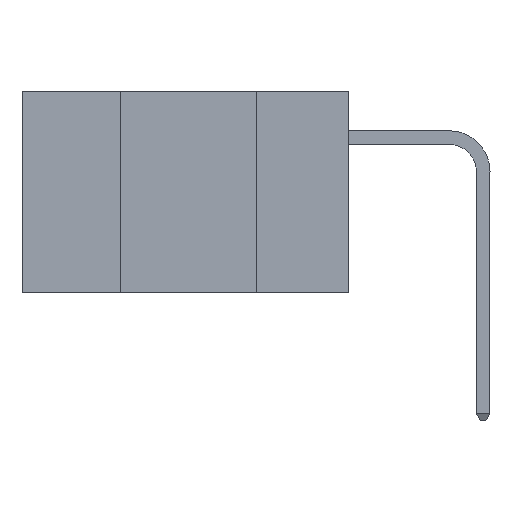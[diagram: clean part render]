
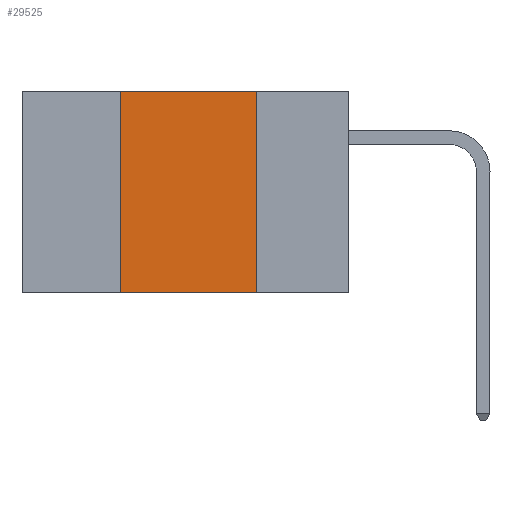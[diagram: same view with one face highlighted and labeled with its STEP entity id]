
A CAD part, left-side view. The second image highlights one B-rep face of the part: STEP entity #29525.
In plain terms, the highlighted planar face has unit normal (-1, 0, 0).
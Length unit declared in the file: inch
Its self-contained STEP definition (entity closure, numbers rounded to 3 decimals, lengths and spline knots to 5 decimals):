
#302 = ORIENTED_EDGE ( 'NONE', *, *, #10548, .T. ) ;
#519 = DIRECTION ( 'NONE',  ( 0., -1., 0. ) ) ;
#1396 = LINE ( 'NONE', #20595, #23088 ) ;
#1943 = VECTOR ( 'NONE', #519, 39.37008 ) ;
#6319 = CARTESIAN_POINT ( 'NONE',  ( 0., 0.42, -0.37 ) ) ;
#9132 = VERTEX_POINT ( 'NONE', #6319 ) ;
#10072 = ORIENTED_EDGE ( 'NONE', *, *, #18065, .F. ) ;
#10548 = EDGE_CURVE ( 'NONE', #9132, #14897, #31810, .T. ) ;
#10995 = CARTESIAN_POINT ( 'NONE',  ( 0., 0.17, 0. ) ) ;
#12280 = DIRECTION ( 'NONE',  ( 0., 0., 1. ) ) ;
#13678 = DIRECTION ( 'NONE',  ( 0., 0., -1. ) ) ;
#14192 = AXIS2_PLACEMENT_3D ( 'NONE', #30654, #25092, #36130 ) ;
#14897 = VERTEX_POINT ( 'NONE', #25280 ) ;
#15468 = DIRECTION ( 'NONE',  ( 0., -1., 0. ) ) ;
#17033 = FACE_OUTER_BOUND ( 'NONE', #19686, .T. ) ;
#18065 = EDGE_CURVE ( 'NONE', #9132, #34963, #1396, .T. ) ;
#18103 = CARTESIAN_POINT ( 'NONE',  ( 0., 0.42, 0. ) ) ;
#19323 = CARTESIAN_POINT ( 'NONE',  ( 0., 0.17, 0. ) ) ;
#19686 = EDGE_LOOP ( 'NONE', ( #31423, #27298, #10072, #302 ) ) ;
#19920 = EDGE_CURVE ( 'NONE', #28088, #14897, #35848, .T. ) ;
#20595 = CARTESIAN_POINT ( 'NONE',  ( 0., 0.42, 0. ) ) ;
#21266 = VECTOR ( 'NONE', #13678, 39.37008 ) ;
#23088 = VECTOR ( 'NONE', #12280, 39.37008 ) ;
#25092 = DIRECTION ( 'NONE',  ( 1., 0., 0. ) ) ;
#25280 = CARTESIAN_POINT ( 'NONE',  ( 0., 0.17, -0.37 ) ) ;
#25847 = CARTESIAN_POINT ( 'NONE',  ( 0., 0.6, -0.37 ) ) ;
#27298 = ORIENTED_EDGE ( 'NONE', *, *, #27555, .F. ) ;
#27555 = EDGE_CURVE ( 'NONE', #34963, #28088, #34861, .T. ) ;
#27572 = VECTOR ( 'NONE', #15468, 39.37008 ) ;
#28088 = VERTEX_POINT ( 'NONE', #10995 ) ;
#29361 = CARTESIAN_POINT ( 'NONE',  ( 0., 0.6, 0. ) ) ;
#29525 = ADVANCED_FACE ( 'NONE', ( #17033 ), #33409, .F. ) ;
#30654 = CARTESIAN_POINT ( 'NONE',  ( 0., 0.6, 0. ) ) ;
#31423 = ORIENTED_EDGE ( 'NONE', *, *, #19920, .F. ) ;
#31810 = LINE ( 'NONE', #25847, #1943 ) ;
#33409 = PLANE ( 'NONE',  #14192 ) ;
#34861 = LINE ( 'NONE', #29361, #27572 ) ;
#34963 = VERTEX_POINT ( 'NONE', #18103 ) ;
#35848 = LINE ( 'NONE', #19323, #21266 ) ;
#36130 = DIRECTION ( 'NONE',  ( 0., 0., -1. ) ) ;
